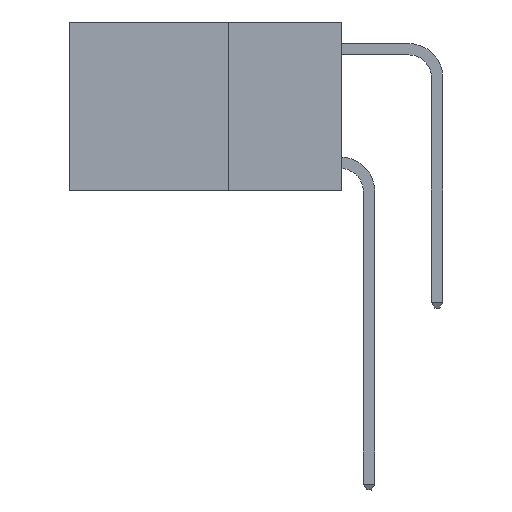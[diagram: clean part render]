
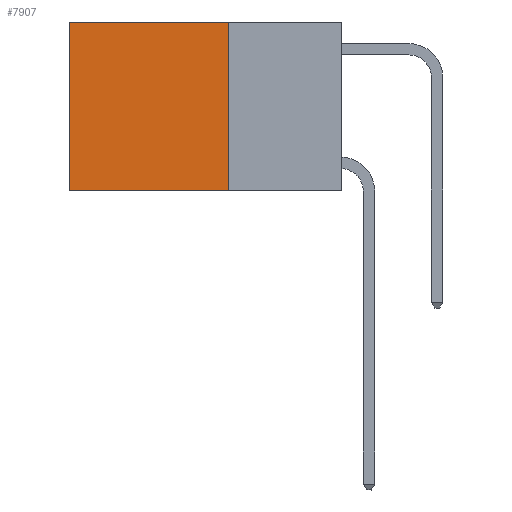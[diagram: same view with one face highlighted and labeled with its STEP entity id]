
A CAD part, left-side view. The second image highlights one B-rep face of the part: STEP entity #7907.
In plain terms, the highlighted planar face has unit normal (-1, 0, 0).
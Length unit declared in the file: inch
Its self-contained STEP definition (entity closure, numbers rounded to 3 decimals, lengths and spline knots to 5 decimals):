
#1626 = CARTESIAN_POINT ( 'NONE',  ( 0.2625, 0.25, 0. ) ) ;
#2031 = CARTESIAN_POINT ( 'NONE',  ( 0.2625, 0.25, 0. ) ) ;
#2081 = LINE ( 'NONE', #6373, #15521 ) ;
#2227 = ORIENTED_EDGE ( 'NONE', *, *, #11799, .F. ) ;
#2549 = VERTEX_POINT ( 'NONE', #8692 ) ;
#3573 = DIRECTION ( 'NONE',  ( 0., 0., -1. ) ) ;
#3817 = EDGE_LOOP ( 'NONE', ( #21291, #14578, #2227, #9190 ) ) ;
#4174 = PLANE ( 'NONE',  #16662 ) ;
#4915 = VECTOR ( 'NONE', #7011, 39.37008 ) ;
#5479 = VERTEX_POINT ( 'NONE', #11177 ) ;
#5942 = DIRECTION ( 'NONE',  ( 0., 0., -1. ) ) ;
#6020 = LINE ( 'NONE', #1626, #15339 ) ;
#6373 = CARTESIAN_POINT ( 'NONE',  ( 0.2625, 0.25, 0. ) ) ;
#7011 = DIRECTION ( 'NONE',  ( 0., 1., 0. ) ) ;
#7459 = FACE_OUTER_BOUND ( 'NONE', #3817, .T. ) ;
#7907 = ADVANCED_FACE ( 'NONE', ( #7459 ), #4174, .F. ) ;
#8692 = CARTESIAN_POINT ( 'NONE',  ( 0.2625, 0.25, -0.37 ) ) ;
#9190 = ORIENTED_EDGE ( 'NONE', *, *, #13797, .T. ) ;
#9617 = LINE ( 'NONE', #22632, #4915 ) ;
#11043 = CARTESIAN_POINT ( 'NONE',  ( 0.2625, 0.25, 0. ) ) ;
#11143 = EDGE_CURVE ( 'NONE', #5479, #15153, #17786, .T. ) ;
#11177 = CARTESIAN_POINT ( 'NONE',  ( 0.2625, 0.6, 0. ) ) ;
#11799 = EDGE_CURVE ( 'NONE', #12931, #2549, #6020, .T. ) ;
#11838 = EDGE_CURVE ( 'NONE', #2549, #15153, #9617, .T. ) ;
#12170 = DIRECTION ( 'NONE',  ( 0., 0., -1. ) ) ;
#12340 = CARTESIAN_POINT ( 'NONE',  ( 0.2625, 0.6, 0. ) ) ;
#12931 = VERTEX_POINT ( 'NONE', #11043 ) ;
#13685 = VECTOR ( 'NONE', #3573, 39.37008 ) ;
#13797 = EDGE_CURVE ( 'NONE', #12931, #5479, #2081, .T. ) ;
#14578 = ORIENTED_EDGE ( 'NONE', *, *, #11838, .F. ) ;
#15153 = VERTEX_POINT ( 'NONE', #22258 ) ;
#15339 = VECTOR ( 'NONE', #12170, 39.37008 ) ;
#15521 = VECTOR ( 'NONE', #16861, 39.37008 ) ;
#16443 = DIRECTION ( 'NONE',  ( 1., 0., 0. ) ) ;
#16662 = AXIS2_PLACEMENT_3D ( 'NONE', #2031, #16443, #5942 ) ;
#16861 = DIRECTION ( 'NONE',  ( 0., 1., 0. ) ) ;
#17786 = LINE ( 'NONE', #12340, #13685 ) ;
#21291 = ORIENTED_EDGE ( 'NONE', *, *, #11143, .T. ) ;
#22258 = CARTESIAN_POINT ( 'NONE',  ( 0.2625, 0.6, -0.37 ) ) ;
#22632 = CARTESIAN_POINT ( 'NONE',  ( 0.2625, 0.25, -0.37 ) ) ;
